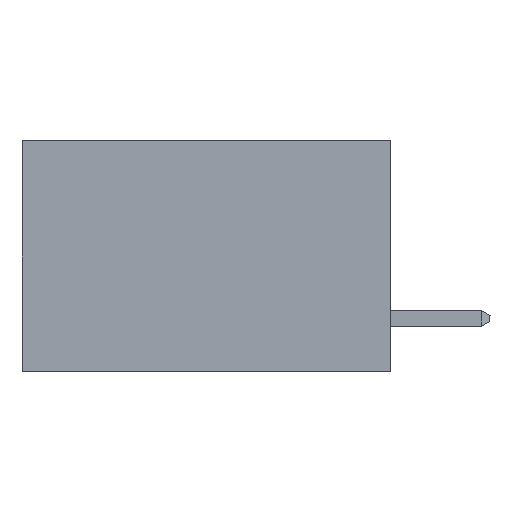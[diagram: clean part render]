
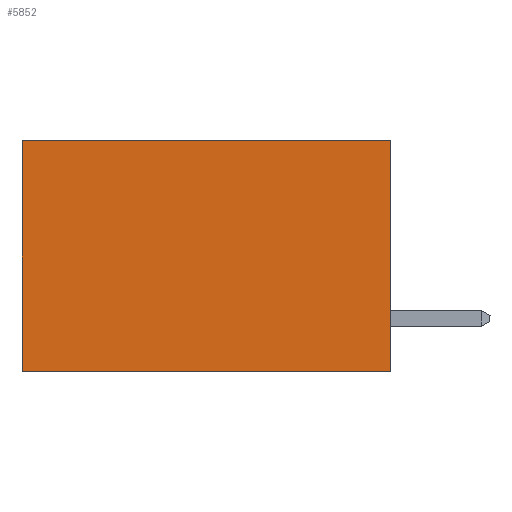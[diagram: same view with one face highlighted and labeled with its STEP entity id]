
A CAD part, left-side view. The second image highlights one B-rep face of the part: STEP entity #5852.
In plain terms, the highlighted planar face has unit normal (-1, 0, 0).
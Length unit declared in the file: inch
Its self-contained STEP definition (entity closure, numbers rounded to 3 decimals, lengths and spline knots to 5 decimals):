
#1107 = EDGE_CURVE ( 'NONE', #27587, #6423, #12160, .T. ) ;
#1572 = ORIENTED_EDGE ( 'NONE', *, *, #14528, .F. ) ;
#1736 = CARTESIAN_POINT ( 'NONE',  ( 0.277, 0.59, -0.37 ) ) ;
#3517 = PLANE ( 'NONE',  #9093 ) ;
#3686 = ORIENTED_EDGE ( 'NONE', *, *, #1107, .F. ) ;
#3767 = EDGE_CURVE ( 'NONE', #6702, #6423, #9818, .T. ) ;
#4558 = DIRECTION ( 'NONE',  ( 0., 0., -1. ) ) ;
#4840 = FACE_OUTER_BOUND ( 'NONE', #8375, .T. ) ;
#5124 = VECTOR ( 'NONE', #14766, 39.37008 ) ;
#5852 = ADVANCED_FACE ( 'NONE', ( #4840 ), #3517, .F. ) ;
#6423 = VERTEX_POINT ( 'NONE', #1736 ) ;
#6702 = VERTEX_POINT ( 'NONE', #13070 ) ;
#8166 = CARTESIAN_POINT ( 'NONE',  ( 0.277, 0., 0. ) ) ;
#8375 = EDGE_LOOP ( 'NONE', ( #9183, #3686, #1572, #16255 ) ) ;
#8575 = DIRECTION ( 'NONE',  ( 0., 0., -1. ) ) ;
#8892 = CARTESIAN_POINT ( 'NONE',  ( 0.277, 0.59, -0.37 ) ) ;
#9059 = VECTOR ( 'NONE', #8575, 39.37008 ) ;
#9093 = AXIS2_PLACEMENT_3D ( 'NONE', #29220, #24173, #25097 ) ;
#9183 = ORIENTED_EDGE ( 'NONE', *, *, #3767, .T. ) ;
#9583 = CARTESIAN_POINT ( 'NONE',  ( 0.277, 0., 0. ) ) ;
#9818 = LINE ( 'NONE', #8892, #9059 ) ;
#9875 = VECTOR ( 'NONE', #4558, 39.37008 ) ;
#10541 = DIRECTION ( 'NONE',  ( 0., 1., 0. ) ) ;
#12160 = LINE ( 'NONE', #14460, #5124 ) ;
#13070 = CARTESIAN_POINT ( 'NONE',  ( 0.277, 0.59, 0. ) ) ;
#14460 = CARTESIAN_POINT ( 'NONE',  ( 0.277, 0., -0.37 ) ) ;
#14528 = EDGE_CURVE ( 'NONE', #15917, #27587, #19259, .T. ) ;
#14766 = DIRECTION ( 'NONE',  ( 0., 1., 0. ) ) ;
#15779 = VECTOR ( 'NONE', #10541, 39.37008 ) ;
#15917 = VERTEX_POINT ( 'NONE', #9583 ) ;
#16255 = ORIENTED_EDGE ( 'NONE', *, *, #18516, .T. ) ;
#18516 = EDGE_CURVE ( 'NONE', #15917, #6702, #27859, .T. ) ;
#18553 = CARTESIAN_POINT ( 'NONE',  ( 0.277, 0., -0.37 ) ) ;
#19259 = LINE ( 'NONE', #18553, #9875 ) ;
#21183 = CARTESIAN_POINT ( 'NONE',  ( 0.277, 0., -0.37 ) ) ;
#24173 = DIRECTION ( 'NONE',  ( 1., 0., 0. ) ) ;
#25097 = DIRECTION ( 'NONE',  ( 0., 0., -1. ) ) ;
#27587 = VERTEX_POINT ( 'NONE', #21183 ) ;
#27859 = LINE ( 'NONE', #8166, #15779 ) ;
#29220 = CARTESIAN_POINT ( 'NONE',  ( 0.277, 0., -0.37 ) ) ;
